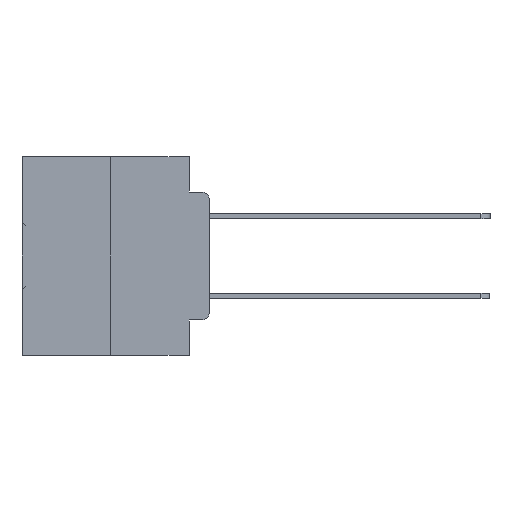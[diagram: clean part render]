
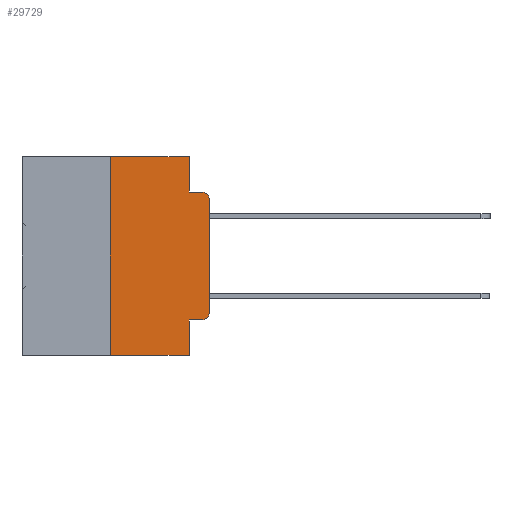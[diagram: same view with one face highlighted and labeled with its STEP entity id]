
A CAD part, left-side view. The second image highlights one B-rep face of the part: STEP entity #29729.
In plain terms, the highlighted planar face has unit normal (-1, 0, 0).
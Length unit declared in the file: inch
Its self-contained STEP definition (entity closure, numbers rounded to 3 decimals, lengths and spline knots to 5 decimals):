
#552 = CARTESIAN_POINT ( 'NONE',  ( 0., 0.02, -0.4115 ) ) ;
#816 = EDGE_CURVE ( 'NONE', #10812, #24489, #34451, .T. ) ;
#1290 = EDGE_CURVE ( 'NONE', #28531, #1508, #13614, .T. ) ;
#1467 = CARTESIAN_POINT ( 'NONE',  ( 0., 0.051, -0.0885 ) ) ;
#1508 = VERTEX_POINT ( 'NONE', #552 ) ;
#1675 = VERTEX_POINT ( 'NONE', #24607 ) ;
#1681 = PLANE ( 'NONE',  #29120 ) ;
#2372 = DIRECTION ( 'NONE',  ( 0., 0., -1. ) ) ;
#2420 = VERTEX_POINT ( 'NONE', #14033 ) ;
#2618 = DIRECTION ( 'NONE',  ( 0., -1., 0. ) ) ;
#2932 = VERTEX_POINT ( 'NONE', #10588 ) ;
#3384 = ORIENTED_EDGE ( 'NONE', *, *, #15669, .F. ) ;
#4195 = LINE ( 'NONE', #20797, #32118 ) ;
#4568 = DIRECTION ( 'NONE',  ( -1., 0., 0. ) ) ;
#4974 = VECTOR ( 'NONE', #20838, 39.37008 ) ;
#5992 = ORIENTED_EDGE ( 'NONE', *, *, #18630, .F. ) ;
#7004 = LINE ( 'NONE', #31263, #20708 ) ;
#7169 = DIRECTION ( 'NONE',  ( 0., 0., 1. ) ) ;
#7312 = DIRECTION ( 'NONE',  ( 0., 0., -1. ) ) ;
#8768 = VECTOR ( 'NONE', #34226, 39.37008 ) ;
#10151 = CARTESIAN_POINT ( 'NONE',  ( 0., 0.473, -0.5 ) ) ;
#10588 = CARTESIAN_POINT ( 'NONE',  ( 0., 0., -0.1085 ) ) ;
#10812 = VERTEX_POINT ( 'NONE', #20243 ) ;
#11432 = EDGE_LOOP ( 'NONE', ( #21788, #17979, #19702, #20537, #22680, #3384, #18018, #5992, #15039, #30122 ) ) ;
#12769 = VECTOR ( 'NONE', #26250, 39.37008 ) ;
#13032 = LINE ( 'NONE', #27670, #26555 ) ;
#13539 = VERTEX_POINT ( 'NONE', #17257 ) ;
#13614 = LINE ( 'NONE', #28738, #12769 ) ;
#14033 = CARTESIAN_POINT ( 'NONE',  ( 0., 0., -0.3915 ) ) ;
#14297 = DIRECTION ( 'NONE',  ( 0., 0., -1. ) ) ;
#14665 = CARTESIAN_POINT ( 'NONE',  ( 0., 0.25, 0. ) ) ;
#14947 = VECTOR ( 'NONE', #20767, 39.37008 ) ;
#15039 = ORIENTED_EDGE ( 'NONE', *, *, #1290, .T. ) ;
#15509 = VERTEX_POINT ( 'NONE', #28336 ) ;
#15669 = EDGE_CURVE ( 'NONE', #15509, #18700, #4195, .T. ) ;
#16084 = LINE ( 'NONE', #10151, #8768 ) ;
#16337 = EDGE_CURVE ( 'NONE', #2932, #13539, #23847, .T. ) ;
#17257 = CARTESIAN_POINT ( 'NONE',  ( 0., 0.02, -0.0885 ) ) ;
#17977 = DIRECTION ( 'NONE',  ( 0., 0., 1. ) ) ;
#17979 = ORIENTED_EDGE ( 'NONE', *, *, #16337, .T. ) ;
#18018 = ORIENTED_EDGE ( 'NONE', *, *, #18280, .T. ) ;
#18280 = EDGE_CURVE ( 'NONE', #15509, #1675, #16084, .T. ) ;
#18630 = EDGE_CURVE ( 'NONE', #28531, #1675, #13032, .T. ) ;
#18700 = VERTEX_POINT ( 'NONE', #14665 ) ;
#18838 = EDGE_CURVE ( 'NONE', #2420, #2932, #7004, .T. ) ;
#18876 = DIRECTION ( 'NONE',  ( -1., 0., 0. ) ) ;
#19114 = CARTESIAN_POINT ( 'NONE',  ( 0., 0.051, -0.0885 ) ) ;
#19702 = ORIENTED_EDGE ( 'NONE', *, *, #25381, .F. ) ;
#20087 = VECTOR ( 'NONE', #2618, 39.37008 ) ;
#20243 = CARTESIAN_POINT ( 'NONE',  ( 0., 0.051, 0. ) ) ;
#20537 = ORIENTED_EDGE ( 'NONE', *, *, #816, .F. ) ;
#20708 = VECTOR ( 'NONE', #17977, 39.37008 ) ;
#20767 = DIRECTION ( 'NONE',  ( 0., -1., 0. ) ) ;
#20797 = CARTESIAN_POINT ( 'NONE',  ( 0., 0.25, 0. ) ) ;
#20801 = CARTESIAN_POINT ( 'NONE',  ( 0., 0.051, 0. ) ) ;
#20838 = DIRECTION ( 'NONE',  ( 0., 0., -1. ) ) ;
#20928 = CARTESIAN_POINT ( 'NONE',  ( 0., 0.473, 0. ) ) ;
#20992 = CARTESIAN_POINT ( 'NONE',  ( 0., 0.02, -0.1085 ) ) ;
#21788 = ORIENTED_EDGE ( 'NONE', *, *, #18838, .T. ) ;
#21908 = EDGE_CURVE ( 'NONE', #18700, #10812, #22164, .T. ) ;
#22164 = LINE ( 'NONE', #34001, #14947 ) ;
#22680 = ORIENTED_EDGE ( 'NONE', *, *, #21908, .F. ) ;
#23649 = DIRECTION ( 'NONE',  ( 1., 0., 0. ) ) ;
#23716 = DIRECTION ( 'NONE',  ( 0., 0., -1. ) ) ;
#23847 = CIRCLE ( 'NONE', #24001, 0.02 ) ;
#24001 = AXIS2_PLACEMENT_3D ( 'NONE', #20992, #4568, #23716 ) ;
#24489 = VERTEX_POINT ( 'NONE', #1467 ) ;
#24607 = CARTESIAN_POINT ( 'NONE',  ( 0., 0.051, -0.5 ) ) ;
#25381 = EDGE_CURVE ( 'NONE', #24489, #13539, #26348, .T. ) ;
#26250 = DIRECTION ( 'NONE',  ( 0., -1., 0. ) ) ;
#26348 = LINE ( 'NONE', #19114, #20087 ) ;
#26555 = VECTOR ( 'NONE', #14297, 39.37008 ) ;
#27670 = CARTESIAN_POINT ( 'NONE',  ( 0., 0.051, 0. ) ) ;
#27973 = CIRCLE ( 'NONE', #28708, 0.02 ) ;
#28336 = CARTESIAN_POINT ( 'NONE',  ( 0., 0.25, -0.5 ) ) ;
#28531 = VERTEX_POINT ( 'NONE', #34580 ) ;
#28708 = AXIS2_PLACEMENT_3D ( 'NONE', #34688, #18876, #2372 ) ;
#28738 = CARTESIAN_POINT ( 'NONE',  ( 0., 0.051, -0.4115 ) ) ;
#29120 = AXIS2_PLACEMENT_3D ( 'NONE', #20928, #23649, #7312 ) ;
#29729 = ADVANCED_FACE ( 'NONE', ( #30632 ), #1681, .F. ) ;
#30122 = ORIENTED_EDGE ( 'NONE', *, *, #31577, .T. ) ;
#30632 = FACE_OUTER_BOUND ( 'NONE', #11432, .T. ) ;
#31263 = CARTESIAN_POINT ( 'NONE',  ( 0., 0., 0. ) ) ;
#31577 = EDGE_CURVE ( 'NONE', #1508, #2420, #27973, .T. ) ;
#32118 = VECTOR ( 'NONE', #7169, 39.37008 ) ;
#34001 = CARTESIAN_POINT ( 'NONE',  ( 0., 0.473, 0. ) ) ;
#34226 = DIRECTION ( 'NONE',  ( 0., -1., 0. ) ) ;
#34451 = LINE ( 'NONE', #20801, #4974 ) ;
#34580 = CARTESIAN_POINT ( 'NONE',  ( 0., 0.051, -0.4115 ) ) ;
#34688 = CARTESIAN_POINT ( 'NONE',  ( 0., 0.02, -0.3915 ) ) ;
